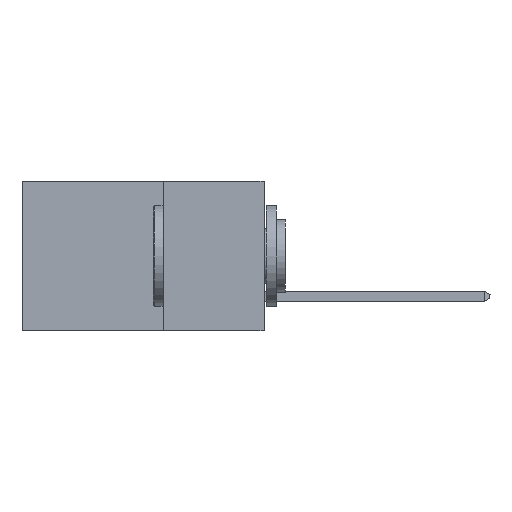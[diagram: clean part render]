
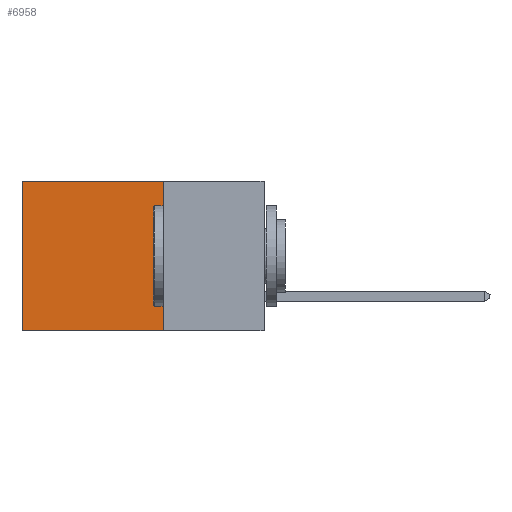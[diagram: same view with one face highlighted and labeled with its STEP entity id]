
A CAD part, left-side view. The second image highlights one B-rep face of the part: STEP entity #6958.
In plain terms, the highlighted planar face has unit normal (-1, 0, 0).
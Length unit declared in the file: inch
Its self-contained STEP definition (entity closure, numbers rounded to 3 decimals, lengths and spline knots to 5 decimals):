
#851 = CARTESIAN_POINT ( 'NONE',  ( 0.2615, 0.25, -0.37 ) ) ;
#1170 = DIRECTION ( 'NONE',  ( 0., 1., 0. ) ) ;
#1206 = VECTOR ( 'NONE', #1170, 39.37008 ) ;
#1286 = ORIENTED_EDGE ( 'NONE', *, *, #9987, .T. ) ;
#1815 = VECTOR ( 'NONE', #6168, 39.37008 ) ;
#2977 = CARTESIAN_POINT ( 'NONE',  ( 0.2615, 0.25, 0. ) ) ;
#3082 = VECTOR ( 'NONE', #4413, 39.37008 ) ;
#3441 = DIRECTION ( 'NONE',  ( 0., 0., -1. ) ) ;
#3773 = FACE_OUTER_BOUND ( 'NONE', #3923, .T. ) ;
#3923 = EDGE_LOOP ( 'NONE', ( #9307, #5487, #3961, #1286 ) ) ;
#3961 = ORIENTED_EDGE ( 'NONE', *, *, #6844, .F. ) ;
#4264 = CARTESIAN_POINT ( 'NONE',  ( 0.2615, 0.25, -0.37 ) ) ;
#4375 = LINE ( 'NONE', #4264, #4862 ) ;
#4413 = DIRECTION ( 'NONE',  ( 0., 0., -1. ) ) ;
#4755 = PLANE ( 'NONE',  #8966 ) ;
#4862 = VECTOR ( 'NONE', #3441, 39.37008 ) ;
#5358 = DIRECTION ( 'NONE',  ( 1., 0., 0. ) ) ;
#5487 = ORIENTED_EDGE ( 'NONE', *, *, #6463, .F. ) ;
#5500 = EDGE_CURVE ( 'NONE', #8926, #6834, #6917, .T. ) ;
#6168 = DIRECTION ( 'NONE',  ( 0., 1., 0. ) ) ;
#6250 = CARTESIAN_POINT ( 'NONE',  ( 0.2615, 0.6, -0.37 ) ) ;
#6463 = EDGE_CURVE ( 'NONE', #9446, #6834, #10234, .T. ) ;
#6834 = VERTEX_POINT ( 'NONE', #10389 ) ;
#6844 = EDGE_CURVE ( 'NONE', #9156, #9446, #4375, .T. ) ;
#6917 = LINE ( 'NONE', #6250, #3082 ) ;
#6958 = ADVANCED_FACE ( 'NONE', ( #3773 ), #4755, .F. ) ;
#7775 = LINE ( 'NONE', #10405, #1815 ) ;
#8729 = CARTESIAN_POINT ( 'NONE',  ( 0.2615, 0.25, -0.37 ) ) ;
#8772 = DIRECTION ( 'NONE',  ( 0., 0., -1. ) ) ;
#8926 = VERTEX_POINT ( 'NONE', #8985 ) ;
#8966 = AXIS2_PLACEMENT_3D ( 'NONE', #9606, #5358, #8772 ) ;
#8985 = CARTESIAN_POINT ( 'NONE',  ( 0.2615, 0.6, 0. ) ) ;
#9156 = VERTEX_POINT ( 'NONE', #2977 ) ;
#9307 = ORIENTED_EDGE ( 'NONE', *, *, #5500, .T. ) ;
#9446 = VERTEX_POINT ( 'NONE', #851 ) ;
#9606 = CARTESIAN_POINT ( 'NONE',  ( 0.2615, 0.25, -0.37 ) ) ;
#9987 = EDGE_CURVE ( 'NONE', #9156, #8926, #7775, .T. ) ;
#10234 = LINE ( 'NONE', #8729, #1206 ) ;
#10389 = CARTESIAN_POINT ( 'NONE',  ( 0.2615, 0.6, -0.37 ) ) ;
#10405 = CARTESIAN_POINT ( 'NONE',  ( 0.2615, 0.25, 0. ) ) ;
